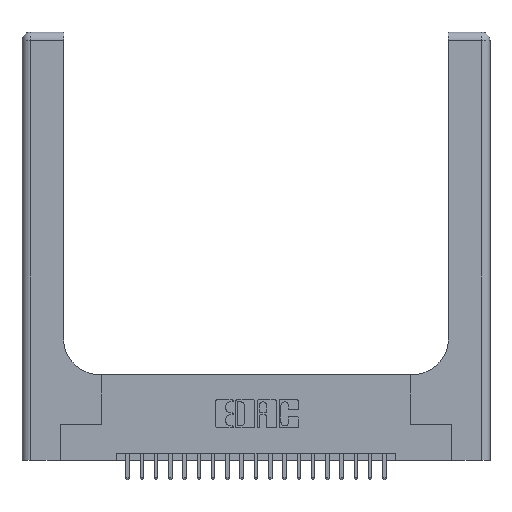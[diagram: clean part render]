
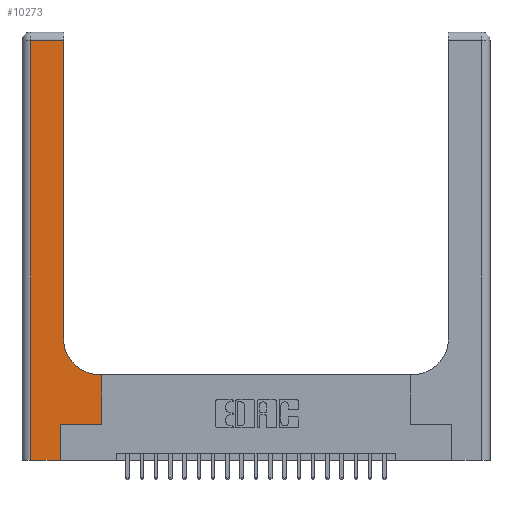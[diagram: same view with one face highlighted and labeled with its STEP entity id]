
A CAD part, top view. The second image highlights one B-rep face of the part: STEP entity #10273.
In plain terms, the highlighted planar face has unit normal (0, 0, 1).
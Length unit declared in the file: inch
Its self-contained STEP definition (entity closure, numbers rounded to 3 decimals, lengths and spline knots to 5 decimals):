
#16 = LINE ( 'NONE', #12048, #835 ) ;
#274 = VECTOR ( 'NONE', #6575, 39.37008 ) ;
#324 = CARTESIAN_POINT ( 'NONE',  ( 0.2915, 0.85, 0.37 ) ) ;
#807 = VERTEX_POINT ( 'NONE', #4236 ) ;
#835 = VECTOR ( 'NONE', #19188, 39.37008 ) ;
#1398 = LINE ( 'NONE', #6886, #21305 ) ;
#1675 = VECTOR ( 'NONE', #16732, 39.37008 ) ;
#1753 = ORIENTED_EDGE ( 'NONE', *, *, #21296, .T. ) ;
#2802 = ORIENTED_EDGE ( 'NONE', *, *, #17067, .T. ) ;
#3327 = VECTOR ( 'NONE', #6619, 39.37008 ) ;
#3816 = VERTEX_POINT ( 'NONE', #324 ) ;
#4059 = AXIS2_PLACEMENT_3D ( 'NONE', #19572, #10532, #15642 ) ;
#4133 = EDGE_CURVE ( 'NONE', #16583, #13108, #16, .T. ) ;
#4236 = CARTESIAN_POINT ( 'NONE',  ( 0.2915, 2.94, 0.37 ) ) ;
#4539 = EDGE_CURVE ( 'NONE', #807, #22659, #6447, .T. ) ;
#4665 = CARTESIAN_POINT ( 'NONE',  ( 0.06, 2.94, 0.37 ) ) ;
#5162 = VERTEX_POINT ( 'NONE', #6907 ) ;
#5302 = CARTESIAN_POINT ( 'NONE',  ( 0.5585, 0.6, 0.37 ) ) ;
#5561 = AXIS2_PLACEMENT_3D ( 'NONE', #17452, #17523, #6805 ) ;
#6447 = LINE ( 'NONE', #21914, #1675 ) ;
#6575 = DIRECTION ( 'NONE',  ( 0., 1., 0. ) ) ;
#6619 = DIRECTION ( 'NONE',  ( 1., 0., 0. ) ) ;
#6692 = DIRECTION ( 'NONE',  ( 0., 1., 0. ) ) ;
#6805 = DIRECTION ( 'NONE',  ( 1., 0., 0. ) ) ;
#6886 = CARTESIAN_POINT ( 'NONE',  ( 0.06, 3., 0.37 ) ) ;
#6907 = CARTESIAN_POINT ( 'NONE',  ( 0.5415, 0.6, 0.37 ) ) ;
#7024 = EDGE_LOOP ( 'NONE', ( #12309, #9471, #13624, #11729, #13392, #10427, #2802, #1753, #17605 ) ) ;
#7420 = EDGE_CURVE ( 'NONE', #22659, #16583, #1398, .T. ) ;
#7448 = EDGE_CURVE ( 'NONE', #3816, #807, #16524, .T. ) ;
#8518 = LINE ( 'NONE', #15831, #19767 ) ;
#8554 = CARTESIAN_POINT ( 'NONE',  ( 0.269, 0.25, 0.37 ) ) ;
#8559 = CIRCLE ( 'NONE', #5561, 0.25 ) ;
#8584 = CARTESIAN_POINT ( 'NONE',  ( 0.2915, 3., 0.37 ) ) ;
#8856 = DIRECTION ( 'NONE',  ( 0., 1., 0. ) ) ;
#9471 = ORIENTED_EDGE ( 'NONE', *, *, #4539, .T. ) ;
#9782 = VECTOR ( 'NONE', #8856, 39.37008 ) ;
#10273 = ADVANCED_FACE ( 'NONE', ( #14747 ), #14004, .F. ) ;
#10274 = EDGE_CURVE ( 'NONE', #5162, #3816, #8559, .T. ) ;
#10427 = ORIENTED_EDGE ( 'NONE', *, *, #20861, .T. ) ;
#10532 = DIRECTION ( 'NONE',  ( 0., 0., -1. ) ) ;
#10687 = CARTESIAN_POINT ( 'NONE',  ( 0.06, 0., 0.37 ) ) ;
#11418 = LINE ( 'NONE', #8554, #3327 ) ;
#11729 = ORIENTED_EDGE ( 'NONE', *, *, #4133, .T. ) ;
#12048 = CARTESIAN_POINT ( 'NONE',  ( 0., 0., 0.37 ) ) ;
#12309 = ORIENTED_EDGE ( 'NONE', *, *, #7448, .T. ) ;
#12703 = VERTEX_POINT ( 'NONE', #5302 ) ;
#13108 = VERTEX_POINT ( 'NONE', #22565 ) ;
#13392 = ORIENTED_EDGE ( 'NONE', *, *, #19784, .T. ) ;
#13435 = LINE ( 'NONE', #16290, #9782 ) ;
#13624 = ORIENTED_EDGE ( 'NONE', *, *, #7420, .T. ) ;
#14004 = PLANE ( 'NONE',  #4059 ) ;
#14747 = FACE_OUTER_BOUND ( 'NONE', #7024, .T. ) ;
#15083 = VECTOR ( 'NONE', #16775, 39.37008 ) ;
#15642 = DIRECTION ( 'NONE',  ( -1., 0., 0. ) ) ;
#15831 = CARTESIAN_POINT ( 'NONE',  ( 0.5585, 0.25, 0.37 ) ) ;
#16286 = VERTEX_POINT ( 'NONE', #17737 ) ;
#16290 = CARTESIAN_POINT ( 'NONE',  ( 0.269, 0., 0.37 ) ) ;
#16524 = LINE ( 'NONE', #8584, #274 ) ;
#16583 = VERTEX_POINT ( 'NONE', #10687 ) ;
#16692 = CARTESIAN_POINT ( 'NONE',  ( 0.2915, 0.6, 0.37 ) ) ;
#16732 = DIRECTION ( 'NONE',  ( -1., 0., 0. ) ) ;
#16775 = DIRECTION ( 'NONE',  ( -1., 0., 0. ) ) ;
#17067 = EDGE_CURVE ( 'NONE', #19343, #12703, #8518, .T. ) ;
#17452 = CARTESIAN_POINT ( 'NONE',  ( 0.5415, 0.85, 0.37 ) ) ;
#17523 = DIRECTION ( 'NONE',  ( 0., 0., -1. ) ) ;
#17605 = ORIENTED_EDGE ( 'NONE', *, *, #10274, .T. ) ;
#17737 = CARTESIAN_POINT ( 'NONE',  ( 0.269, 0.25, 0.37 ) ) ;
#18170 = LINE ( 'NONE', #16692, #15083 ) ;
#19188 = DIRECTION ( 'NONE',  ( 1., 0., 0. ) ) ;
#19343 = VERTEX_POINT ( 'NONE', #23066 ) ;
#19572 = CARTESIAN_POINT ( 'NONE',  ( 0., 3., 0.37 ) ) ;
#19767 = VECTOR ( 'NONE', #6692, 39.37008 ) ;
#19784 = EDGE_CURVE ( 'NONE', #13108, #16286, #13435, .T. ) ;
#20861 = EDGE_CURVE ( 'NONE', #16286, #19343, #11418, .T. ) ;
#21216 = DIRECTION ( 'NONE',  ( 0., -1., 0. ) ) ;
#21296 = EDGE_CURVE ( 'NONE', #12703, #5162, #18170, .T. ) ;
#21305 = VECTOR ( 'NONE', #21216, 39.37008 ) ;
#21914 = CARTESIAN_POINT ( 'NONE',  ( 0., 2.94, 0.37 ) ) ;
#22565 = CARTESIAN_POINT ( 'NONE',  ( 0.269, 0., 0.37 ) ) ;
#22659 = VERTEX_POINT ( 'NONE', #4665 ) ;
#23066 = CARTESIAN_POINT ( 'NONE',  ( 0.5585, 0.25, 0.37 ) ) ;
